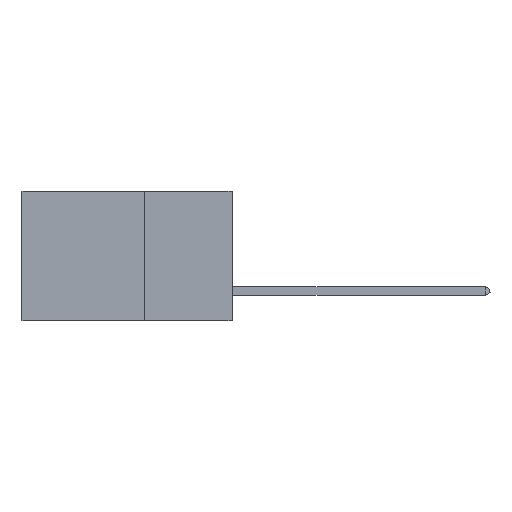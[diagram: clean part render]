
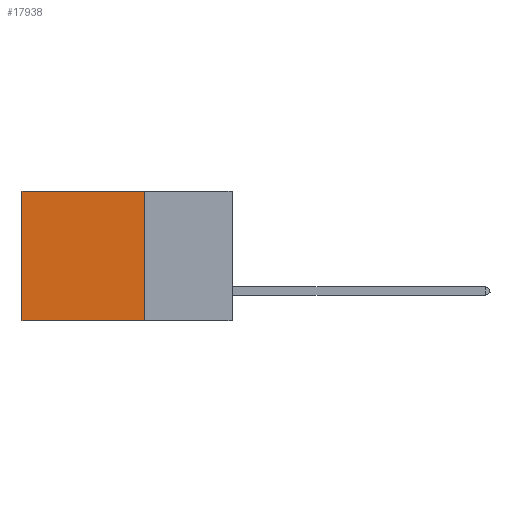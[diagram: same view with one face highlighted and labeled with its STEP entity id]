
A CAD part, left-side view. The second image highlights one B-rep face of the part: STEP entity #17938.
In plain terms, the highlighted planar face has unit normal (-1, 0, 0).
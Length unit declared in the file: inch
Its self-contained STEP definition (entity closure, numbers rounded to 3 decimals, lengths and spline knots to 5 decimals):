
#255 = LINE ( 'NONE', #10504, #20069 ) ;
#544 = EDGE_CURVE ( 'NONE', #11498, #17138, #255, .T. ) ;
#707 = VERTEX_POINT ( 'NONE', #14341 ) ;
#2398 = DIRECTION ( 'NONE',  ( 0., 1., 0. ) ) ;
#2422 = CARTESIAN_POINT ( 'NONE',  ( 0.2875, 0.6, 0. ) ) ;
#3641 = EDGE_CURVE ( 'NONE', #14254, #17138, #17394, .T. ) ;
#3855 = DIRECTION ( 'NONE',  ( 0., 0., -1. ) ) ;
#4818 = LINE ( 'NONE', #6992, #9511 ) ;
#5458 = CARTESIAN_POINT ( 'NONE',  ( 0.2875, 0.25, 0. ) ) ;
#5659 = AXIS2_PLACEMENT_3D ( 'NONE', #9070, #13582, #20131 ) ;
#6224 = ORIENTED_EDGE ( 'NONE', *, *, #544, .F. ) ;
#6382 = EDGE_CURVE ( 'NONE', #707, #14254, #10337, .T. ) ;
#6992 = CARTESIAN_POINT ( 'NONE',  ( 0.2875, 0.25, 0. ) ) ;
#7421 = CARTESIAN_POINT ( 'NONE',  ( 0.2875, 0.6, -0.37 ) ) ;
#7489 = PLANE ( 'NONE',  #5659 ) ;
#7770 = FACE_OUTER_BOUND ( 'NONE', #14157, .T. ) ;
#9019 = ORIENTED_EDGE ( 'NONE', *, *, #3641, .T. ) ;
#9070 = CARTESIAN_POINT ( 'NONE',  ( 0.2875, 0.25, 0. ) ) ;
#9511 = VECTOR ( 'NONE', #3855, 39.37008 ) ;
#10337 = LINE ( 'NONE', #5458, #12598 ) ;
#10504 = CARTESIAN_POINT ( 'NONE',  ( 0.2875, 0.25, -0.37 ) ) ;
#11032 = EDGE_CURVE ( 'NONE', #707, #11498, #4818, .T. ) ;
#11498 = VERTEX_POINT ( 'NONE', #12264 ) ;
#11627 = DIRECTION ( 'NONE',  ( 0., 1., 0. ) ) ;
#12264 = CARTESIAN_POINT ( 'NONE',  ( 0.2875, 0.25, -0.37 ) ) ;
#12289 = DIRECTION ( 'NONE',  ( 0., 0., -1. ) ) ;
#12598 = VECTOR ( 'NONE', #11627, 39.37008 ) ;
#13286 = ORIENTED_EDGE ( 'NONE', *, *, #11032, .F. ) ;
#13404 = VECTOR ( 'NONE', #12289, 39.37008 ) ;
#13582 = DIRECTION ( 'NONE',  ( 1., 0., 0. ) ) ;
#13740 = CARTESIAN_POINT ( 'NONE',  ( 0.2875, 0.6, 0. ) ) ;
#14157 = EDGE_LOOP ( 'NONE', ( #9019, #6224, #13286, #17327 ) ) ;
#14254 = VERTEX_POINT ( 'NONE', #2422 ) ;
#14341 = CARTESIAN_POINT ( 'NONE',  ( 0.2875, 0.25, 0. ) ) ;
#17138 = VERTEX_POINT ( 'NONE', #7421 ) ;
#17327 = ORIENTED_EDGE ( 'NONE', *, *, #6382, .T. ) ;
#17394 = LINE ( 'NONE', #13740, #13404 ) ;
#17938 = ADVANCED_FACE ( 'NONE', ( #7770 ), #7489, .F. ) ;
#20069 = VECTOR ( 'NONE', #2398, 39.37008 ) ;
#20131 = DIRECTION ( 'NONE',  ( 0., 0., -1. ) ) ;
